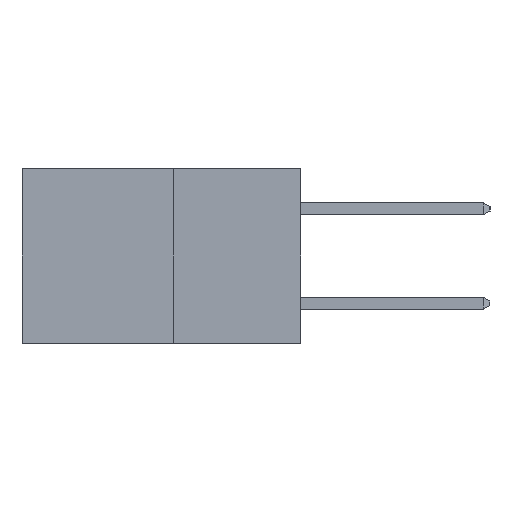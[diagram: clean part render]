
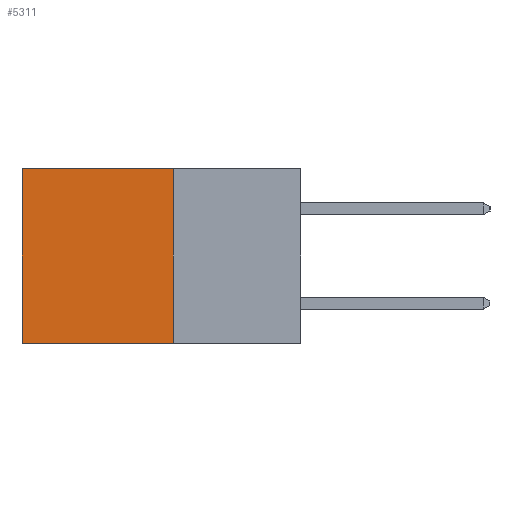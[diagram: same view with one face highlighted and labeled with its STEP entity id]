
A CAD part, left-side view. The second image highlights one B-rep face of the part: STEP entity #5311.
In plain terms, the highlighted planar face has unit normal (-1, 0, 0).
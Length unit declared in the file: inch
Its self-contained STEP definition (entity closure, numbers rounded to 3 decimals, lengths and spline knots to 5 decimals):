
#836 = ORIENTED_EDGE ( 'NONE', *, *, #9799, .F. ) ;
#2179 = DIRECTION ( 'NONE',  ( 0., 0., -1. ) ) ;
#2181 = VECTOR ( 'NONE', #18520, 39.37008 ) ;
#3030 = LINE ( 'NONE', #13201, #20620 ) ;
#3157 = DIRECTION ( 'NONE',  ( 0., 0., -1. ) ) ;
#4575 = EDGE_CURVE ( 'NONE', #20390, #16469, #10224, .T. ) ;
#4984 = VECTOR ( 'NONE', #11429, 39.37008 ) ;
#5311 = ADVANCED_FACE ( 'NONE', ( #18121 ), #20339, .F. ) ;
#5406 = EDGE_LOOP ( 'NONE', ( #21141, #5985, #836, #12268 ) ) ;
#5985 = ORIENTED_EDGE ( 'NONE', *, *, #4575, .F. ) ;
#7587 = AXIS2_PLACEMENT_3D ( 'NONE', #10566, #12216, #2179 ) ;
#7627 = EDGE_CURVE ( 'NONE', #19702, #19934, #13867, .T. ) ;
#8619 = CARTESIAN_POINT ( 'NONE',  ( 0.277, 0.27, 0. ) ) ;
#9799 = EDGE_CURVE ( 'NONE', #19702, #20390, #3030, .T. ) ;
#10224 = LINE ( 'NONE', #14092, #18418 ) ;
#10566 = CARTESIAN_POINT ( 'NONE',  ( 0.277, 0.27, -0.37 ) ) ;
#11125 = LINE ( 'NONE', #20207, #2181 ) ;
#11429 = DIRECTION ( 'NONE',  ( 0., 1., 0. ) ) ;
#11486 = EDGE_CURVE ( 'NONE', #19934, #16469, #11125, .T. ) ;
#12216 = DIRECTION ( 'NONE',  ( 1., 0., 0. ) ) ;
#12239 = CARTESIAN_POINT ( 'NONE',  ( 0.277, 0.27, -0.37 ) ) ;
#12268 = ORIENTED_EDGE ( 'NONE', *, *, #7627, .T. ) ;
#12473 = CARTESIAN_POINT ( 'NONE',  ( 0.277, 0.59, 0. ) ) ;
#13201 = CARTESIAN_POINT ( 'NONE',  ( 0.277, 0.27, -0.37 ) ) ;
#13867 = LINE ( 'NONE', #19481, #4984 ) ;
#13882 = DIRECTION ( 'NONE',  ( 0., 1., 0. ) ) ;
#14092 = CARTESIAN_POINT ( 'NONE',  ( 0.277, 0.27, -0.37 ) ) ;
#16469 = VERTEX_POINT ( 'NONE', #19022 ) ;
#18121 = FACE_OUTER_BOUND ( 'NONE', #5406, .T. ) ;
#18418 = VECTOR ( 'NONE', #13882, 39.37008 ) ;
#18520 = DIRECTION ( 'NONE',  ( 0., 0., -1. ) ) ;
#19022 = CARTESIAN_POINT ( 'NONE',  ( 0.277, 0.59, -0.37 ) ) ;
#19481 = CARTESIAN_POINT ( 'NONE',  ( 0.277, 0.27, 0. ) ) ;
#19702 = VERTEX_POINT ( 'NONE', #8619 ) ;
#19934 = VERTEX_POINT ( 'NONE', #12473 ) ;
#20207 = CARTESIAN_POINT ( 'NONE',  ( 0.277, 0.59, -0.37 ) ) ;
#20339 = PLANE ( 'NONE',  #7587 ) ;
#20390 = VERTEX_POINT ( 'NONE', #12239 ) ;
#20620 = VECTOR ( 'NONE', #3157, 39.37008 ) ;
#21141 = ORIENTED_EDGE ( 'NONE', *, *, #11486, .T. ) ;
